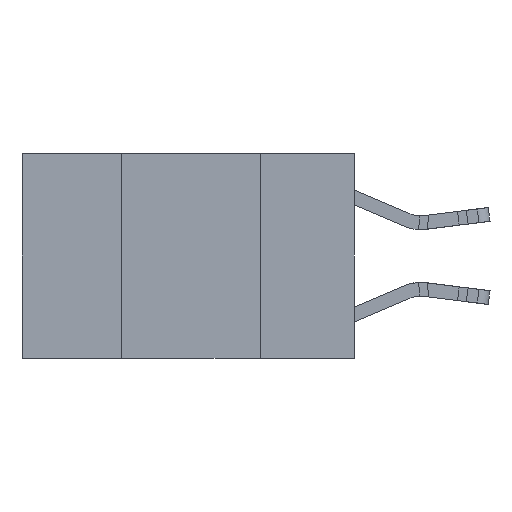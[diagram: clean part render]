
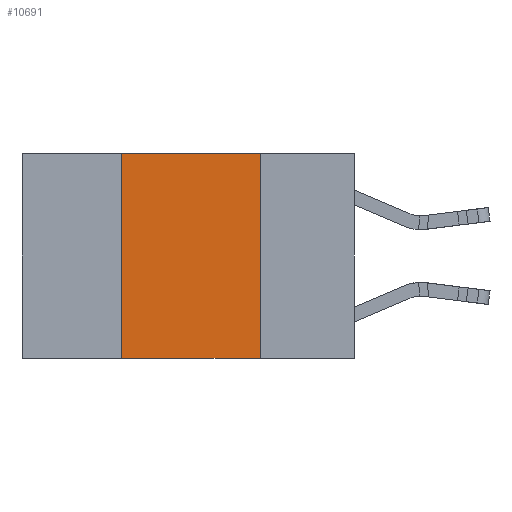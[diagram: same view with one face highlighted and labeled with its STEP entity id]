
A CAD part, left-side view. The second image highlights one B-rep face of the part: STEP entity #10691.
In plain terms, the highlighted planar face has unit normal (-1, 0, 0).
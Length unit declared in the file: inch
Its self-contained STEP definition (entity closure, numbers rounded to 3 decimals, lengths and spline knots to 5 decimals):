
#394 = DIRECTION ( 'NONE',  ( 0., -1., 0. ) ) ;
#593 = CARTESIAN_POINT ( 'NONE',  ( 0., 0.42, 0. ) ) ;
#640 = LINE ( 'NONE', #15465, #2886 ) ;
#1844 = DIRECTION ( 'NONE',  ( 0., 0., -1. ) ) ;
#2146 = AXIS2_PLACEMENT_3D ( 'NONE', #5160, #7650, #16721 ) ;
#2886 = VECTOR ( 'NONE', #8431, 39.37008 ) ;
#3569 = VERTEX_POINT ( 'NONE', #5876 ) ;
#4482 = LINE ( 'NONE', #11663, #30246 ) ;
#5160 = CARTESIAN_POINT ( 'NONE',  ( 0., 0.6, 0. ) ) ;
#5876 = CARTESIAN_POINT ( 'NONE',  ( 0., 0.17, 0. ) ) ;
#6200 = ORIENTED_EDGE ( 'NONE', *, *, #13130, .F. ) ;
#7196 = PLANE ( 'NONE',  #2146 ) ;
#7650 = DIRECTION ( 'NONE',  ( 1., 0., 0. ) ) ;
#8431 = DIRECTION ( 'NONE',  ( 0., 0., 1. ) ) ;
#9808 = ORIENTED_EDGE ( 'NONE', *, *, #18750, .T. ) ;
#10691 = ADVANCED_FACE ( 'NONE', ( #28642 ), #7196, .F. ) ;
#11013 = EDGE_CURVE ( 'NONE', #3569, #19396, #30328, .T. ) ;
#11663 = CARTESIAN_POINT ( 'NONE',  ( 0., 0.6, 0. ) ) ;
#11690 = CARTESIAN_POINT ( 'NONE',  ( 0., 0.17, 0. ) ) ;
#11750 = VERTEX_POINT ( 'NONE', #593 ) ;
#12283 = VECTOR ( 'NONE', #1844, 39.37008 ) ;
#13130 = EDGE_CURVE ( 'NONE', #17978, #11750, #640, .T. ) ;
#13616 = CARTESIAN_POINT ( 'NONE',  ( 0., 0.17, -0.37 ) ) ;
#14611 = DIRECTION ( 'NONE',  ( 0., -1., 0. ) ) ;
#15465 = CARTESIAN_POINT ( 'NONE',  ( 0., 0.42, 0. ) ) ;
#15755 = CARTESIAN_POINT ( 'NONE',  ( 0., 0.42, -0.37 ) ) ;
#16115 = EDGE_LOOP ( 'NONE', ( #19180, #24834, #6200, #9808 ) ) ;
#16721 = DIRECTION ( 'NONE',  ( 0., 0., -1. ) ) ;
#17626 = VECTOR ( 'NONE', #14611, 39.37008 ) ;
#17978 = VERTEX_POINT ( 'NONE', #15755 ) ;
#18750 = EDGE_CURVE ( 'NONE', #17978, #19396, #26214, .T. ) ;
#19180 = ORIENTED_EDGE ( 'NONE', *, *, #11013, .F. ) ;
#19396 = VERTEX_POINT ( 'NONE', #13616 ) ;
#21165 = EDGE_CURVE ( 'NONE', #11750, #3569, #4482, .T. ) ;
#21532 = CARTESIAN_POINT ( 'NONE',  ( 0., 0.6, -0.37 ) ) ;
#24834 = ORIENTED_EDGE ( 'NONE', *, *, #21165, .F. ) ;
#26214 = LINE ( 'NONE', #21532, #17626 ) ;
#28642 = FACE_OUTER_BOUND ( 'NONE', #16115, .T. ) ;
#30246 = VECTOR ( 'NONE', #394, 39.37008 ) ;
#30328 = LINE ( 'NONE', #11690, #12283 ) ;
